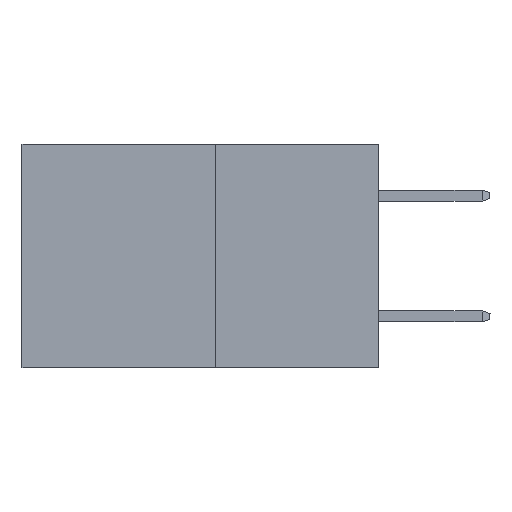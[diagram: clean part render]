
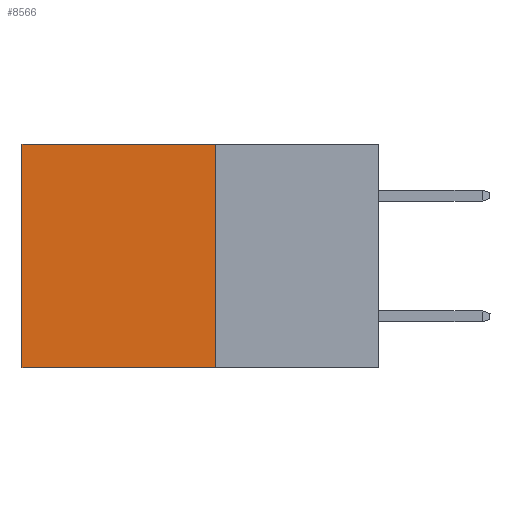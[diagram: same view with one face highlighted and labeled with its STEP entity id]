
A CAD part, left-side view. The second image highlights one B-rep face of the part: STEP entity #8566.
In plain terms, the highlighted planar face has unit normal (-1, 0, 0).
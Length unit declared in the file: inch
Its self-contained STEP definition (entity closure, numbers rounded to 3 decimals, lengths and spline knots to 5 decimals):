
#396 = VERTEX_POINT ( 'NONE', #15244 ) ;
#770 = EDGE_CURVE ( 'NONE', #19819, #3660, #847, .T. ) ;
#847 = LINE ( 'NONE', #11641, #13485 ) ;
#916 = DIRECTION ( 'NONE',  ( 0., 0., -1. ) ) ;
#2106 = VECTOR ( 'NONE', #916, 39.37008 ) ;
#2693 = CARTESIAN_POINT ( 'NONE',  ( 0.277, 0.27, 0. ) ) ;
#3170 = CARTESIAN_POINT ( 'NONE',  ( 0.277, 0.59, -0.37 ) ) ;
#3575 = CARTESIAN_POINT ( 'NONE',  ( 0.277, 0.27, -0.37 ) ) ;
#3660 = VERTEX_POINT ( 'NONE', #7512 ) ;
#3861 = DIRECTION ( 'NONE',  ( 1., 0., 0. ) ) ;
#4859 = DIRECTION ( 'NONE',  ( 0., 0., -1. ) ) ;
#5667 = ORIENTED_EDGE ( 'NONE', *, *, #770, .F. ) ;
#5812 = CARTESIAN_POINT ( 'NONE',  ( 0.277, 0.27, -0.37 ) ) ;
#7073 = CARTESIAN_POINT ( 'NONE',  ( 0.277, 0.27, 0. ) ) ;
#7512 = CARTESIAN_POINT ( 'NONE',  ( 0.277, 0.59, -0.37 ) ) ;
#8566 = ADVANCED_FACE ( 'NONE', ( #12015 ), #13744, .F. ) ;
#8790 = CARTESIAN_POINT ( 'NONE',  ( 0.277, 0.27, -0.37 ) ) ;
#9362 = VECTOR ( 'NONE', #14222, 39.37008 ) ;
#10053 = EDGE_LOOP ( 'NONE', ( #16061, #5667, #17926, #13664 ) ) ;
#10507 = DIRECTION ( 'NONE',  ( 0., 1., 0. ) ) ;
#10833 = LINE ( 'NONE', #3170, #14101 ) ;
#10882 = EDGE_CURVE ( 'NONE', #17771, #396, #16947, .T. ) ;
#11641 = CARTESIAN_POINT ( 'NONE',  ( 0.277, 0.27, -0.37 ) ) ;
#12015 = FACE_OUTER_BOUND ( 'NONE', #10053, .T. ) ;
#13485 = VECTOR ( 'NONE', #10507, 39.37008 ) ;
#13664 = ORIENTED_EDGE ( 'NONE', *, *, #10882, .T. ) ;
#13744 = PLANE ( 'NONE',  #14129 ) ;
#14101 = VECTOR ( 'NONE', #4859, 39.37008 ) ;
#14129 = AXIS2_PLACEMENT_3D ( 'NONE', #8790, #3861, #15338 ) ;
#14222 = DIRECTION ( 'NONE',  ( 0., 1., 0. ) ) ;
#14698 = LINE ( 'NONE', #5812, #2106 ) ;
#15244 = CARTESIAN_POINT ( 'NONE',  ( 0.277, 0.59, 0. ) ) ;
#15338 = DIRECTION ( 'NONE',  ( 0., 0., -1. ) ) ;
#16061 = ORIENTED_EDGE ( 'NONE', *, *, #16791, .T. ) ;
#16791 = EDGE_CURVE ( 'NONE', #396, #3660, #10833, .T. ) ;
#16947 = LINE ( 'NONE', #2693, #9362 ) ;
#17771 = VERTEX_POINT ( 'NONE', #7073 ) ;
#17926 = ORIENTED_EDGE ( 'NONE', *, *, #20071, .F. ) ;
#19819 = VERTEX_POINT ( 'NONE', #3575 ) ;
#20071 = EDGE_CURVE ( 'NONE', #17771, #19819, #14698, .T. ) ;
